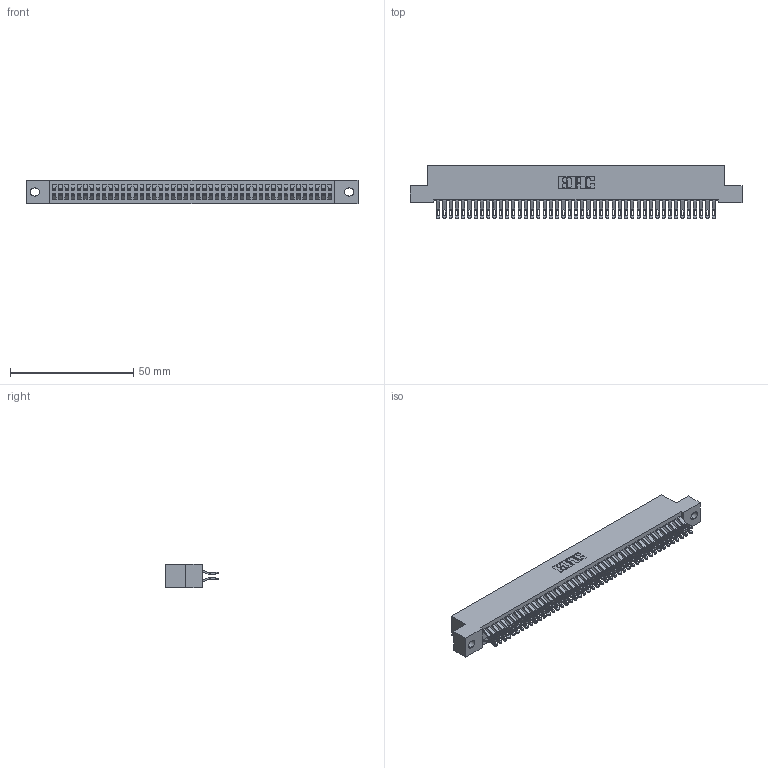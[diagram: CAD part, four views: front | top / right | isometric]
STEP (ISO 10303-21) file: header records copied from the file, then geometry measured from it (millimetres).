
FILE_DESCRIPTION (( 'STEP AP203' ), '1' );
FILE_NAME ('342-090-555-202.STEP', '2019-10-04T14:23:56', ( '' ), ( '' ), 'SwSTEP 2.0', 'SolidWorks 2016', '' );
FILE_SCHEMA (( 'CONFIG_CONTROL_DESIGN' ));
Length unit declared in the file: inch
Products named in the file (3): 342-090-555-202; 342 Part_.128 Slot; 345-292-001_555 Tail
Assembly tree (91 placements, depth 2):
  342-090-555-202
    342 Part_.128 Slot
    345-292-001_555 Tail  x90
Bounding box: 134.62 x 21.47 x 9.4 mm (x, y, z)
Volume: 12307.8 mm3; surface area: 20738.2 mm2
Topology: 91 solids, 91 shells, 5334 faces, 16781 edges, 11186 vertices
Faces by surface type: plane 3130, cylinder 2204
Entity records: 28891 total; most frequent: CARTESIAN_POINT 4820, ORIENTED_EDGE 4726, DIRECTION 4083, EDGE_CURVE 2363, VECTOR 2215, LINE 2215, VERTEX_POINT 1574, AXIS2_PLACEMENT_3D 934
